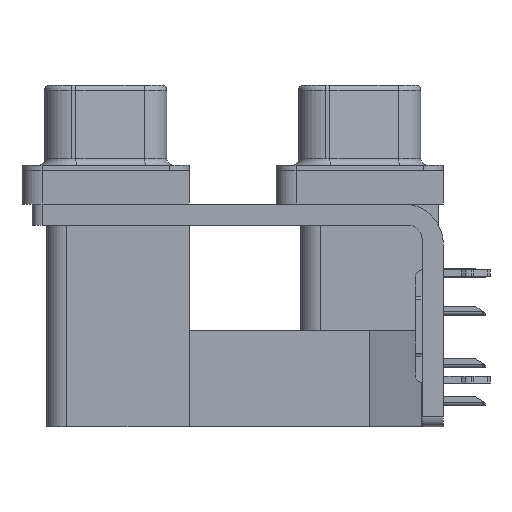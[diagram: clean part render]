
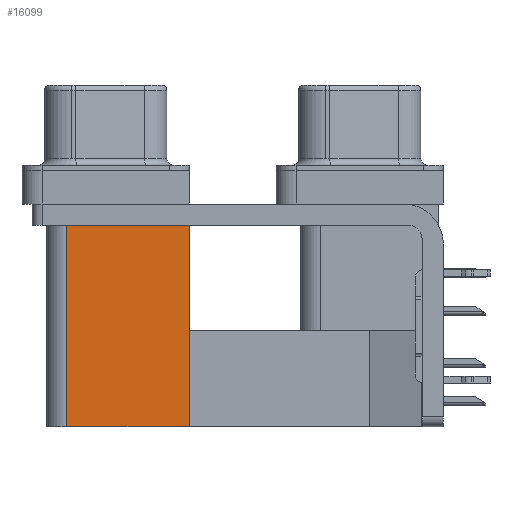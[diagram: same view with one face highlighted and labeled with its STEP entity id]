
A CAD part, left-side view. The second image highlights one B-rep face of the part: STEP entity #16099.
In plain terms, the highlighted planar face has unit normal (-1, 0, 0).
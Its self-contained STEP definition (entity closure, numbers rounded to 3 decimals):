
#737 = VERTEX_POINT ( 'NONE', #15581 ) ;
#1325 = LINE ( 'NONE', #14148, #12684 ) ;
#2071 = LINE ( 'NONE', #8530, #2797 ) ;
#2797 = VECTOR ( 'NONE', #6668, 1000. ) ;
#3312 = LINE ( 'NONE', #12102, #11987 ) ;
#3819 = EDGE_LOOP ( 'NONE', ( #19028, #4984, #7521, #24746 ) ) ;
#4984 = ORIENTED_EDGE ( 'NONE', *, *, #8952, .F. ) ;
#6564 = FACE_OUTER_BOUND ( 'NONE', #3819, .T. ) ;
#6668 = DIRECTION ( 'NONE',  ( 0., 0., 1. ) ) ;
#7521 = ORIENTED_EDGE ( 'NONE', *, *, #19440, .F. ) ;
#7598 = CARTESIAN_POINT ( 'NONE',  ( 3.79, 21.975, -2.5 ) ) ;
#8530 = CARTESIAN_POINT ( 'NONE',  ( 3.79, 12.775, -19.2 ) ) ;
#8712 = DIRECTION ( 'NONE',  ( 1., 0., 0. ) ) ;
#8952 = EDGE_CURVE ( 'NONE', #28345, #14225, #3312, .T. ) ;
#9715 = LINE ( 'NONE', #17019, #20078 ) ;
#10094 = DIRECTION ( 'NONE',  ( 0., 1., 0. ) ) ;
#11987 = VECTOR ( 'NONE', #15826, 1000. ) ;
#12102 = CARTESIAN_POINT ( 'NONE',  ( 3.79, 21.975, -19.2 ) ) ;
#12684 = VECTOR ( 'NONE', #10094, 1000. ) ;
#13337 = CARTESIAN_POINT ( 'NONE',  ( 3.79, 21.975, -19.2 ) ) ;
#14148 = CARTESIAN_POINT ( 'NONE',  ( 3.79, 12.775, -2.5 ) ) ;
#14225 = VERTEX_POINT ( 'NONE', #7598 ) ;
#15341 = PLANE ( 'NONE',  #17938 ) ;
#15581 = CARTESIAN_POINT ( 'NONE',  ( 3.79, 12.775, -19.2 ) ) ;
#15826 = DIRECTION ( 'NONE',  ( 0., 0., 1. ) ) ;
#16099 = ADVANCED_FACE ( 'NONE', ( #6564 ), #15341, .F. ) ;
#16737 = DIRECTION ( 'NONE',  ( 0., 1., 0. ) ) ;
#17019 = CARTESIAN_POINT ( 'NONE',  ( 3.79, 12.775, -19.2 ) ) ;
#17489 = DIRECTION ( 'NONE',  ( 0., 1., 0. ) ) ;
#17938 = AXIS2_PLACEMENT_3D ( 'NONE', #22377, #8712, #17489 ) ;
#18710 = EDGE_CURVE ( 'NONE', #27852, #14225, #1325, .T. ) ;
#19028 = ORIENTED_EDGE ( 'NONE', *, *, #18710, .T. ) ;
#19440 = EDGE_CURVE ( 'NONE', #737, #28345, #9715, .T. ) ;
#20078 = VECTOR ( 'NONE', #16737, 1000. ) ;
#21037 = EDGE_CURVE ( 'NONE', #737, #27852, #2071, .T. ) ;
#22377 = CARTESIAN_POINT ( 'NONE',  ( 3.79, 12.775, -19.2 ) ) ;
#24746 = ORIENTED_EDGE ( 'NONE', *, *, #21037, .T. ) ;
#27353 = CARTESIAN_POINT ( 'NONE',  ( 3.79, 12.775, -2.5 ) ) ;
#27852 = VERTEX_POINT ( 'NONE', #27353 ) ;
#28345 = VERTEX_POINT ( 'NONE', #13337 ) ;
